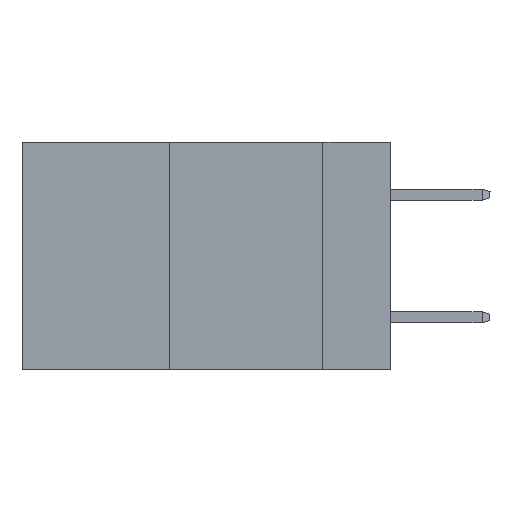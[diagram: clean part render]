
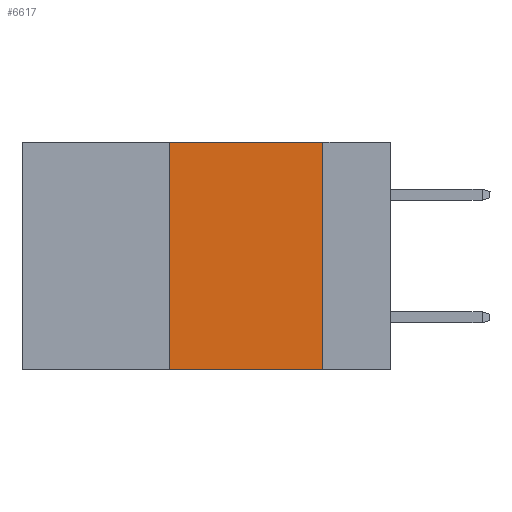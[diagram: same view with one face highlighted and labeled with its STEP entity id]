
A CAD part, left-side view. The second image highlights one B-rep face of the part: STEP entity #6617.
In plain terms, the highlighted planar face has unit normal (-1, 0, 0).
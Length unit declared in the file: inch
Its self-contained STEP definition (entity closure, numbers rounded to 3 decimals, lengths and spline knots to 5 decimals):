
#237 = ORIENTED_EDGE ( 'NONE', *, *, #9784, .F. ) ;
#1278 = CARTESIAN_POINT ( 'NONE',  ( 0., 0.6, -0.37 ) ) ;
#1432 = VERTEX_POINT ( 'NONE', #10278 ) ;
#1952 = CARTESIAN_POINT ( 'NONE',  ( 0., 0.11, 0. ) ) ;
#2017 = DIRECTION ( 'NONE',  ( 0., -1., 0. ) ) ;
#2207 = CARTESIAN_POINT ( 'NONE',  ( 0., 0.6, 0. ) ) ;
#4715 = PLANE ( 'NONE',  #16609 ) ;
#5517 = ORIENTED_EDGE ( 'NONE', *, *, #16292, .F. ) ;
#6134 = CARTESIAN_POINT ( 'NONE',  ( 0., 0.6, 0. ) ) ;
#6617 = ADVANCED_FACE ( 'NONE', ( #15739 ), #4715, .F. ) ;
#6765 = CARTESIAN_POINT ( 'NONE',  ( 0., 0.36, -0.37 ) ) ;
#6874 = LINE ( 'NONE', #1278, #13672 ) ;
#7923 = EDGE_CURVE ( 'NONE', #11801, #17833, #12862, .T. ) ;
#8152 = DIRECTION ( 'NONE',  ( 0., 0., -1. ) ) ;
#8437 = CARTESIAN_POINT ( 'NONE',  ( 0., 0.36, 0. ) ) ;
#8549 = VECTOR ( 'NONE', #8152, 39.37008 ) ;
#8687 = DIRECTION ( 'NONE',  ( 1., 0., 0. ) ) ;
#8918 = EDGE_CURVE ( 'NONE', #11801, #1432, #6874, .T. ) ;
#9784 = EDGE_CURVE ( 'NONE', #17833, #10989, #10560, .T. ) ;
#10278 = CARTESIAN_POINT ( 'NONE',  ( 0., 0.11, -0.37 ) ) ;
#10362 = ORIENTED_EDGE ( 'NONE', *, *, #8918, .T. ) ;
#10560 = LINE ( 'NONE', #2207, #17551 ) ;
#10711 = DIRECTION ( 'NONE',  ( 0., 0., 1. ) ) ;
#10859 = ORIENTED_EDGE ( 'NONE', *, *, #7923, .F. ) ;
#10989 = VERTEX_POINT ( 'NONE', #1952 ) ;
#11801 = VERTEX_POINT ( 'NONE', #6765 ) ;
#12124 = CARTESIAN_POINT ( 'NONE',  ( 0., 0.36, 0. ) ) ;
#12652 = EDGE_LOOP ( 'NONE', ( #5517, #237, #10859, #10362 ) ) ;
#12862 = LINE ( 'NONE', #12124, #17666 ) ;
#13672 = VECTOR ( 'NONE', #16527, 39.37008 ) ;
#14042 = LINE ( 'NONE', #17834, #8549 ) ;
#15726 = DIRECTION ( 'NONE',  ( 0., 0., -1. ) ) ;
#15739 = FACE_OUTER_BOUND ( 'NONE', #12652, .T. ) ;
#16292 = EDGE_CURVE ( 'NONE', #10989, #1432, #14042, .T. ) ;
#16527 = DIRECTION ( 'NONE',  ( 0., -1., 0. ) ) ;
#16609 = AXIS2_PLACEMENT_3D ( 'NONE', #6134, #8687, #15726 ) ;
#17551 = VECTOR ( 'NONE', #2017, 39.37008 ) ;
#17666 = VECTOR ( 'NONE', #10711, 39.37008 ) ;
#17833 = VERTEX_POINT ( 'NONE', #8437 ) ;
#17834 = CARTESIAN_POINT ( 'NONE',  ( 0., 0.11, 0. ) ) ;
